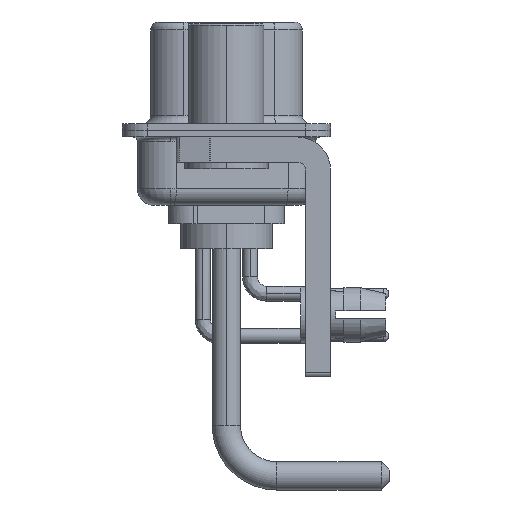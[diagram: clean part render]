
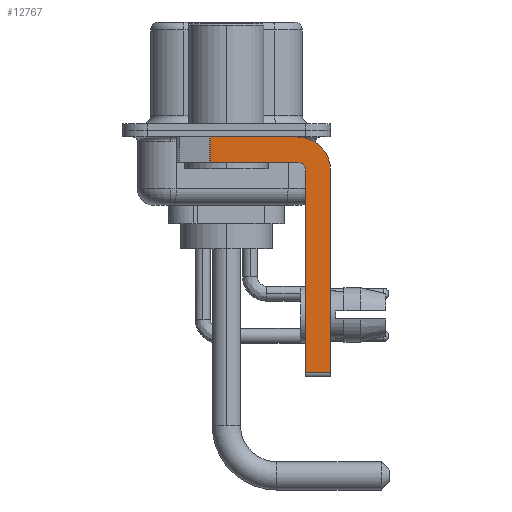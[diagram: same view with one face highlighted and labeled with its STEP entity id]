
A CAD part, left-side view. The second image highlights one B-rep face of the part: STEP entity #12767.
In plain terms, the highlighted planar face has unit normal (-1, 0, 0).
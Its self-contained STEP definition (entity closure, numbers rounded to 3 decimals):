
#344 = VERTEX_POINT ( 'NONE', #14644 ) ;
#461 = EDGE_CURVE ( 'NONE', #15562, #10984, #29038, .T. ) ;
#837 = DIRECTION ( 'NONE',  ( 0., 0., -1. ) ) ;
#932 = CARTESIAN_POINT ( 'NONE',  ( -2.9, 0.978, -0.4 ) ) ;
#1348 = AXIS2_PLACEMENT_3D ( 'NONE', #27870, #25569, #4590 ) ;
#1513 = CARTESIAN_POINT ( 'NONE',  ( -2.9, -6.25, -14.55 ) ) ;
#2080 = DIRECTION ( 'NONE',  ( 1., 0., 0. ) ) ;
#3046 = LINE ( 'NONE', #17313, #5725 ) ;
#3367 = EDGE_CURVE ( 'NONE', #344, #10984, #20576, .T. ) ;
#3541 = VERTEX_POINT ( 'NONE', #19028 ) ;
#4482 = CARTESIAN_POINT ( 'NONE',  ( -2.9, -4.25, -1.9 ) ) ;
#4590 = DIRECTION ( 'NONE',  ( 0., 0., 1. ) ) ;
#5611 = VERTEX_POINT ( 'NONE', #18747 ) ;
#5725 = VECTOR ( 'NONE', #5840, 1000. ) ;
#5840 = DIRECTION ( 'NONE',  ( 0., -1., 0. ) ) ;
#6320 = AXIS2_PLACEMENT_3D ( 'NONE', #25575, #13961, #23441 ) ;
#6622 = DIRECTION ( 'NONE',  ( 0., -1., 0. ) ) ;
#6838 = EDGE_CURVE ( 'NONE', #3541, #24848, #8712, .T. ) ;
#6897 = DIRECTION ( 'NONE',  ( 0., 0., 1. ) ) ;
#7316 = EDGE_LOOP ( 'NONE', ( #11675, #20937, #26530, #17389, #21303, #27498, #23822, #11618 ) ) ;
#7517 = EDGE_CURVE ( 'NONE', #15562, #11186, #29587, .T. ) ;
#8712 = LINE ( 'NONE', #27208, #22379 ) ;
#10984 = VERTEX_POINT ( 'NONE', #11531 ) ;
#11102 = DIRECTION ( 'NONE',  ( 0., 1., 0. ) ) ;
#11186 = VERTEX_POINT ( 'NONE', #13344 ) ;
#11475 = AXIS2_PLACEMENT_3D ( 'NONE', #18345, #2080, #24926 ) ;
#11493 = LINE ( 'NONE', #11806, #12526 ) ;
#11531 = CARTESIAN_POINT ( 'NONE',  ( -2.9, 0.978, -1.9 ) ) ;
#11618 = ORIENTED_EDGE ( 'NONE', *, *, #28785, .F. ) ;
#11675 = ORIENTED_EDGE ( 'NONE', *, *, #7517, .F. ) ;
#11806 = CARTESIAN_POINT ( 'NONE',  ( -2.9, -4.75, -14.8 ) ) ;
#12526 = VECTOR ( 'NONE', #6897, 1000. ) ;
#12767 = ADVANCED_FACE ( 'NONE', ( #13463 ), #16187, .F. ) ;
#13344 = CARTESIAN_POINT ( 'NONE',  ( -2.9, -4.25, -0.4 ) ) ;
#13463 = FACE_OUTER_BOUND ( 'NONE', #7316, .T. ) ;
#13725 = VECTOR ( 'NONE', #11102, 1000. ) ;
#13961 = DIRECTION ( 'NONE',  ( 1., 0., 0. ) ) ;
#14644 = CARTESIAN_POINT ( 'NONE',  ( -2.9, -4.25, -1.9 ) ) ;
#14907 = VECTOR ( 'NONE', #6622, 1000. ) ;
#15064 = CARTESIAN_POINT ( 'NONE',  ( -2.9, -4.75, -2.4 ) ) ;
#15562 = VERTEX_POINT ( 'NONE', #932 ) ;
#16187 = PLANE ( 'NONE',  #11475 ) ;
#16866 = VERTEX_POINT ( 'NONE', #15064 ) ;
#17313 = CARTESIAN_POINT ( 'NONE',  ( -2.9, -4.25, -14.55 ) ) ;
#17389 = ORIENTED_EDGE ( 'NONE', *, *, #27423, .F. ) ;
#17949 = EDGE_CURVE ( 'NONE', #5611, #24848, #3046, .T. ) ;
#18345 = CARTESIAN_POINT ( 'NONE',  ( -2.9, -4.25, -2.4 ) ) ;
#18747 = CARTESIAN_POINT ( 'NONE',  ( -2.9, -4.75, -14.55 ) ) ;
#19028 = CARTESIAN_POINT ( 'NONE',  ( -2.9, -6.25, -2.4 ) ) ;
#20576 = LINE ( 'NONE', #4482, #13725 ) ;
#20937 = ORIENTED_EDGE ( 'NONE', *, *, #461, .T. ) ;
#21303 = ORIENTED_EDGE ( 'NONE', *, *, #25072, .F. ) ;
#22379 = VECTOR ( 'NONE', #22770, 1000. ) ;
#22770 = DIRECTION ( 'NONE',  ( 0., 0., -1. ) ) ;
#23441 = DIRECTION ( 'NONE',  ( 0., 0., -1. ) ) ;
#23760 = VECTOR ( 'NONE', #837, 1000. ) ;
#23822 = ORIENTED_EDGE ( 'NONE', *, *, #6838, .F. ) ;
#23920 = CIRCLE ( 'NONE', #6320, 2. ) ;
#24848 = VERTEX_POINT ( 'NONE', #1513 ) ;
#24926 = DIRECTION ( 'NONE',  ( 0., 0., -1. ) ) ;
#25072 = EDGE_CURVE ( 'NONE', #5611, #16866, #11493, .T. ) ;
#25569 = DIRECTION ( 'NONE',  ( -1., 0., 0. ) ) ;
#25575 = CARTESIAN_POINT ( 'NONE',  ( -2.9, -4.25, -2.4 ) ) ;
#26530 = ORIENTED_EDGE ( 'NONE', *, *, #3367, .F. ) ;
#26738 = CARTESIAN_POINT ( 'NONE',  ( -2.9, 0.978, -1.9 ) ) ;
#27208 = CARTESIAN_POINT ( 'NONE',  ( -2.9, -6.25, -2.4 ) ) ;
#27423 = EDGE_CURVE ( 'NONE', #16866, #344, #27768, .T. ) ;
#27498 = ORIENTED_EDGE ( 'NONE', *, *, #17949, .T. ) ;
#27569 = CARTESIAN_POINT ( 'NONE',  ( -2.9, 3., -0.4 ) ) ;
#27768 = CIRCLE ( 'NONE', #1348, 0.5 ) ;
#27870 = CARTESIAN_POINT ( 'NONE',  ( -2.9, -4.25, -2.4 ) ) ;
#28785 = EDGE_CURVE ( 'NONE', #11186, #3541, #23920, .T. ) ;
#29038 = LINE ( 'NONE', #26738, #23760 ) ;
#29587 = LINE ( 'NONE', #27569, #14907 ) ;
